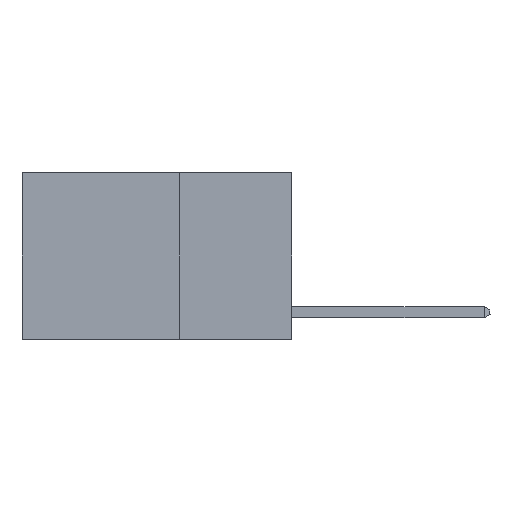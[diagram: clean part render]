
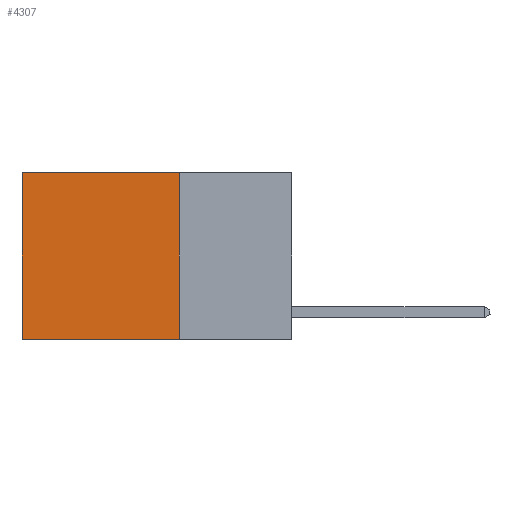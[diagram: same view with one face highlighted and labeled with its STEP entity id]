
A CAD part, left-side view. The second image highlights one B-rep face of the part: STEP entity #4307.
In plain terms, the highlighted planar face has unit normal (-1, 0, 0).
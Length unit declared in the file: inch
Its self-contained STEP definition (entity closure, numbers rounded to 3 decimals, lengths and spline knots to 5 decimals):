
#152 = ORIENTED_EDGE ( 'NONE', *, *, #1949, .F. ) ;
#734 = DIRECTION ( 'NONE',  ( 0., 1., 0. ) ) ;
#1039 = LINE ( 'NONE', #11506, #9335 ) ;
#1237 = CARTESIAN_POINT ( 'NONE',  ( 0.2625, 0.6, 0. ) ) ;
#1949 = EDGE_CURVE ( 'NONE', #7339, #4635, #6467, .T. ) ;
#2042 = DIRECTION ( 'NONE',  ( 0., 0., -1. ) ) ;
#2043 = VERTEX_POINT ( 'NONE', #3719 ) ;
#2418 = EDGE_CURVE ( 'NONE', #12189, #4635, #1039, .T. ) ;
#3555 = VECTOR ( 'NONE', #10690, 39.37008 ) ;
#3719 = CARTESIAN_POINT ( 'NONE',  ( 0.2625, 0.25, 0. ) ) ;
#4307 = ADVANCED_FACE ( 'NONE', ( #13742 ), #7403, .F. ) ;
#4635 = VERTEX_POINT ( 'NONE', #6838 ) ;
#5270 = EDGE_LOOP ( 'NONE', ( #8449, #152, #8803, #11609 ) ) ;
#6332 = CARTESIAN_POINT ( 'NONE',  ( 0.2625, 0.25, 0. ) ) ;
#6467 = LINE ( 'NONE', #11078, #3555 ) ;
#6838 = CARTESIAN_POINT ( 'NONE',  ( 0.2625, 0.6, -0.37 ) ) ;
#7339 = VERTEX_POINT ( 'NONE', #11262 ) ;
#7403 = PLANE ( 'NONE',  #13409 ) ;
#8449 = ORIENTED_EDGE ( 'NONE', *, *, #2418, .T. ) ;
#8511 = DIRECTION ( 'NONE',  ( 1., 0., 0. ) ) ;
#8803 = ORIENTED_EDGE ( 'NONE', *, *, #12762, .F. ) ;
#9335 = VECTOR ( 'NONE', #11454, 39.37008 ) ;
#9431 = VECTOR ( 'NONE', #734, 39.37008 ) ;
#9999 = CARTESIAN_POINT ( 'NONE',  ( 0.2625, 0.25, 0. ) ) ;
#10119 = LINE ( 'NONE', #13608, #9431 ) ;
#10690 = DIRECTION ( 'NONE',  ( 0., 1., 0. ) ) ;
#11045 = DIRECTION ( 'NONE',  ( 0., 0., -1. ) ) ;
#11078 = CARTESIAN_POINT ( 'NONE',  ( 0.2625, 0.25, -0.37 ) ) ;
#11262 = CARTESIAN_POINT ( 'NONE',  ( 0.2625, 0.25, -0.37 ) ) ;
#11454 = DIRECTION ( 'NONE',  ( 0., 0., -1. ) ) ;
#11506 = CARTESIAN_POINT ( 'NONE',  ( 0.2625, 0.6, 0. ) ) ;
#11609 = ORIENTED_EDGE ( 'NONE', *, *, #13654, .T. ) ;
#11736 = VECTOR ( 'NONE', #11045, 39.37008 ) ;
#12068 = LINE ( 'NONE', #9999, #11736 ) ;
#12189 = VERTEX_POINT ( 'NONE', #1237 ) ;
#12762 = EDGE_CURVE ( 'NONE', #2043, #7339, #12068, .T. ) ;
#13409 = AXIS2_PLACEMENT_3D ( 'NONE', #6332, #8511, #2042 ) ;
#13608 = CARTESIAN_POINT ( 'NONE',  ( 0.2625, 0.25, 0. ) ) ;
#13654 = EDGE_CURVE ( 'NONE', #2043, #12189, #10119, .T. ) ;
#13742 = FACE_OUTER_BOUND ( 'NONE', #5270, .T. ) ;
